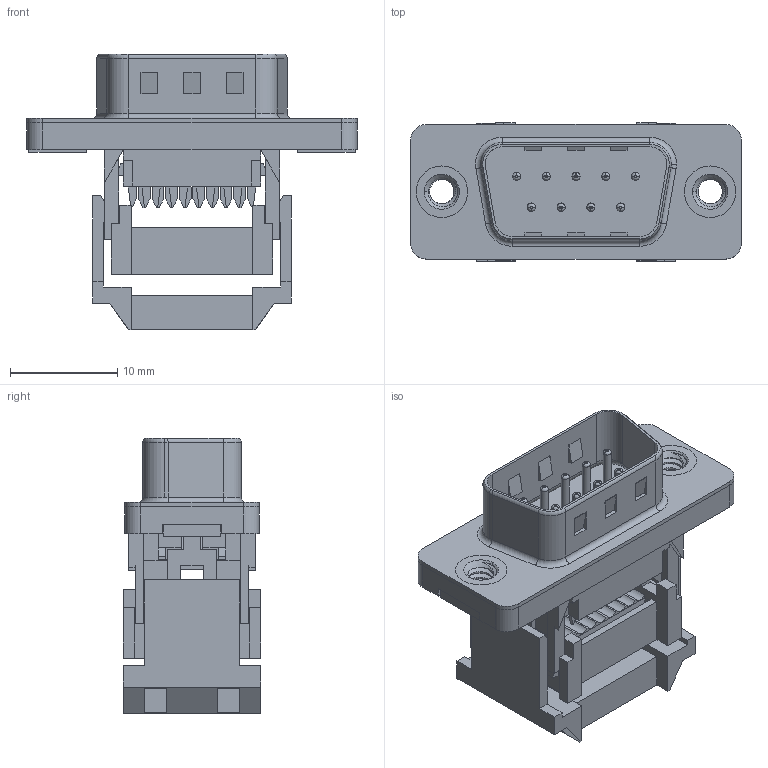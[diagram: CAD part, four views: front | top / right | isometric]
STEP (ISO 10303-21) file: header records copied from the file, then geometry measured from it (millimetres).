
FILE_DESCRIPTION (( 'STEP AP203' ), '1' );
FILE_NAME ('627-009-227-212.STEP', '2020-07-16T13:57:02', ( '' ), ( '' ), 'SwSTEP 2.0', 'SolidWorks 2020', '' );
FILE_SCHEMA (( 'CONFIG_CONTROL_DESIGN' ));
Length unit declared in the file: millimetre
Products named in the file (8): 627 IDC Cable Cover_09 Contacts; 627 PB Shell_09 Contacts; 627-009-227-212; 627 IDC Contacts_09 Contacts; 627 IDC Guide Front_09 Contacts; 627 IDC 4-40 Threaded Rivet; 627 IDC Guide Rear_09 Contacts; 627 IDC Housing_09 Contacts
Assembly tree (8 placements, depth 2):
  627-009-227-212
    627 IDC Housing_09 Contacts
    627 PB Shell_09 Contacts
    627 IDC Contacts_09 Contacts
    627 IDC Guide Front_09 Contacts
    627 IDC Guide Rear_09 Contacts
    627 IDC Cable Cover_09 Contacts
    627 IDC 4-40 Threaded Rivet  x2
Bounding box: 30.81 x 12.85 x 25.7 mm (x, y, z)
Volume: 2773.5 mm3; surface area: 5937.6 mm2
Topology: 18 solids, 18 shells, 1168 faces, 3196 edges, 2077 vertices
Faces by surface type: plane 855, cylinder 251, torus 46, cone 10, bspline 6
Entity records: 38022 total; most frequent: CARTESIAN_POINT 7740, ORIENTED_EDGE 6242, DIRECTION 5959, EDGE_CURVE 3121, LINE 2519, VECTOR 2519, VERTEX_POINT 2028, AXIS2_PLACEMENT_3D 1720
